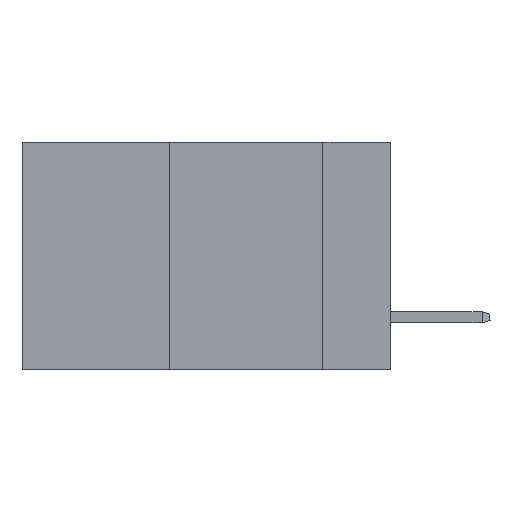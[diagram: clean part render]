
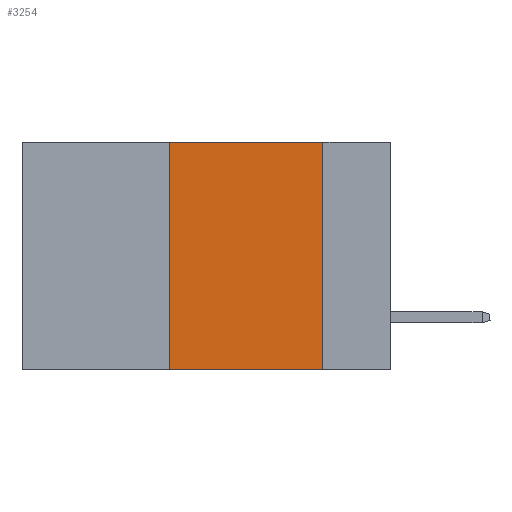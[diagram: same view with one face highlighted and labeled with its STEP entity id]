
A CAD part, left-side view. The second image highlights one B-rep face of the part: STEP entity #3254.
In plain terms, the highlighted planar face has unit normal (-1, 0, 0).
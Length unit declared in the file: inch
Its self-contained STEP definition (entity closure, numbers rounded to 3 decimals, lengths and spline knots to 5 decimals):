
#361 = VERTEX_POINT ( 'NONE', #10908 ) ;
#487 = EDGE_CURVE ( 'NONE', #15731, #17317, #15777, .T. ) ;
#571 = AXIS2_PLACEMENT_3D ( 'NONE', #9638, #15239, #13905 ) ;
#993 = VECTOR ( 'NONE', #16884, 39.37008 ) ;
#2628 = CARTESIAN_POINT ( 'NONE',  ( 0., 0.6, 0. ) ) ;
#2836 = ORIENTED_EDGE ( 'NONE', *, *, #6629, .T. ) ;
#3254 = ADVANCED_FACE ( 'NONE', ( #17961 ), #5104, .F. ) ;
#3437 = VECTOR ( 'NONE', #14276, 39.37008 ) ;
#4217 = LINE ( 'NONE', #5270, #993 ) ;
#4616 = LINE ( 'NONE', #11753, #12982 ) ;
#5104 = PLANE ( 'NONE',  #571 ) ;
#5270 = CARTESIAN_POINT ( 'NONE',  ( 0., 0.36, 0. ) ) ;
#5935 = EDGE_CURVE ( 'NONE', #17317, #13213, #4616, .T. ) ;
#6629 = EDGE_CURVE ( 'NONE', #361, #13213, #6822, .T. ) ;
#6822 = LINE ( 'NONE', #8494, #3437 ) ;
#6871 = DIRECTION ( 'NONE',  ( 0., -1., 0. ) ) ;
#7394 = EDGE_LOOP ( 'NONE', ( #15342, #10560, #15383, #2836 ) ) ;
#8494 = CARTESIAN_POINT ( 'NONE',  ( 0., 0.6, -0.37 ) ) ;
#9638 = CARTESIAN_POINT ( 'NONE',  ( 0., 0.6, 0. ) ) ;
#10560 = ORIENTED_EDGE ( 'NONE', *, *, #487, .F. ) ;
#10908 = CARTESIAN_POINT ( 'NONE',  ( 0., 0.36, -0.37 ) ) ;
#11753 = CARTESIAN_POINT ( 'NONE',  ( 0., 0.11, 0. ) ) ;
#12982 = VECTOR ( 'NONE', #16088, 39.37008 ) ;
#13213 = VERTEX_POINT ( 'NONE', #17781 ) ;
#13853 = CARTESIAN_POINT ( 'NONE',  ( 0., 0.11, 0. ) ) ;
#13905 = DIRECTION ( 'NONE',  ( 0., 0., -1. ) ) ;
#13987 = VECTOR ( 'NONE', #6871, 39.37008 ) ;
#14276 = DIRECTION ( 'NONE',  ( 0., -1., 0. ) ) ;
#15239 = DIRECTION ( 'NONE',  ( 1., 0., 0. ) ) ;
#15342 = ORIENTED_EDGE ( 'NONE', *, *, #5935, .F. ) ;
#15383 = ORIENTED_EDGE ( 'NONE', *, *, #18213, .F. ) ;
#15712 = CARTESIAN_POINT ( 'NONE',  ( 0., 0.36, 0. ) ) ;
#15731 = VERTEX_POINT ( 'NONE', #15712 ) ;
#15777 = LINE ( 'NONE', #2628, #13987 ) ;
#16088 = DIRECTION ( 'NONE',  ( 0., 0., -1. ) ) ;
#16884 = DIRECTION ( 'NONE',  ( 0., 0., 1. ) ) ;
#17317 = VERTEX_POINT ( 'NONE', #13853 ) ;
#17781 = CARTESIAN_POINT ( 'NONE',  ( 0., 0.11, -0.37 ) ) ;
#17961 = FACE_OUTER_BOUND ( 'NONE', #7394, .T. ) ;
#18213 = EDGE_CURVE ( 'NONE', #361, #15731, #4217, .T. ) ;
